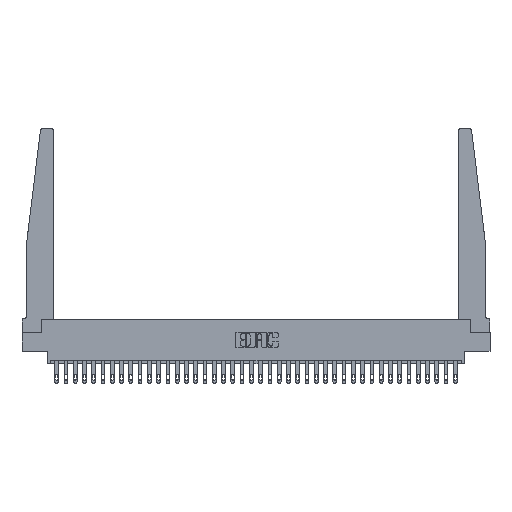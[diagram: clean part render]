
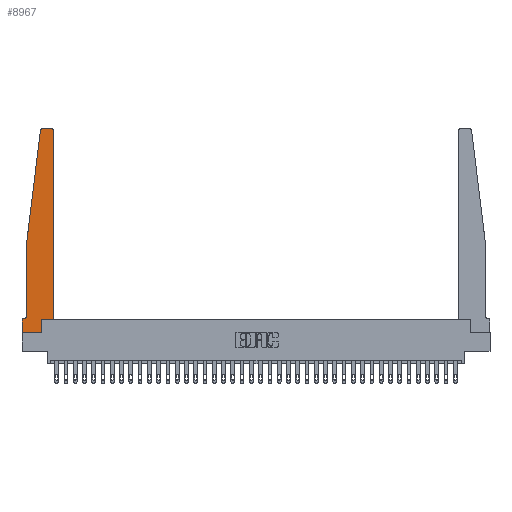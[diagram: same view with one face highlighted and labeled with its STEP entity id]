
A CAD part, top view. The second image highlights one B-rep face of the part: STEP entity #8967.
In plain terms, the highlighted planar face has unit normal (0, 0, 1).
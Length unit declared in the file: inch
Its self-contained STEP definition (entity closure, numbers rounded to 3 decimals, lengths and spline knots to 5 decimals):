
#457 = ORIENTED_EDGE ( 'NONE', *, *, #11465, .T. ) ;
#671 = ORIENTED_EDGE ( 'NONE', *, *, #31473, .T. ) ;
#787 = VERTEX_POINT ( 'NONE', #23877 ) ;
#1664 = VECTOR ( 'NONE', #19332, 39.37008 ) ;
#2096 = VERTEX_POINT ( 'NONE', #30226 ) ;
#2302 = DIRECTION ( 'NONE',  ( 1., 0., 0. ) ) ;
#2799 = DIRECTION ( 'NONE',  ( 0., 0., -1. ) ) ;
#3092 = LINE ( 'NONE', #8354, #9274 ) ;
#3141 = EDGE_CURVE ( 'NONE', #31485, #24207, #18799, .T. ) ;
#4517 = AXIS2_PLACEMENT_3D ( 'NONE', #7769, #13542, #21088 ) ;
#4764 = AXIS2_PLACEMENT_3D ( 'NONE', #23436, #2799, #31823 ) ;
#5004 = VECTOR ( 'NONE', #18298, 39.37008 ) ;
#5695 = EDGE_CURVE ( 'NONE', #9499, #8446, #24652, .T. ) ;
#5712 = VERTEX_POINT ( 'NONE', #26736 ) ;
#5932 = LINE ( 'NONE', #10493, #8910 ) ;
#6143 = VECTOR ( 'NONE', #16947, 39.37008 ) ;
#6240 = CARTESIAN_POINT ( 'NONE',  ( 0.065, 1.25, 0.37 ) ) ;
#6490 = LINE ( 'NONE', #16515, #27529 ) ;
#7472 = CARTESIAN_POINT ( 'NONE',  ( 0.25, 2.75, 0.37 ) ) ;
#7582 = LINE ( 'NONE', #13000, #5004 ) ;
#7655 = EDGE_CURVE ( 'NONE', #25096, #787, #6490, .T. ) ;
#7769 = CARTESIAN_POINT ( 'NONE',  ( 0.395, 2.72, 0.37 ) ) ;
#8354 = CARTESIAN_POINT ( 'NONE',  ( 0.065, 0.1875, 0.37 ) ) ;
#8446 = VERTEX_POINT ( 'NONE', #28793 ) ;
#8910 = VECTOR ( 'NONE', #31875, 39.37008 ) ;
#8967 = ADVANCED_FACE ( 'NONE', ( #17964 ), #18292, .T. ) ;
#9274 = VECTOR ( 'NONE', #31438, 39.37008 ) ;
#9285 = ORIENTED_EDGE ( 'NONE', *, *, #10119, .T. ) ;
#9445 = VERTEX_POINT ( 'NONE', #16657 ) ;
#9499 = VERTEX_POINT ( 'NONE', #13752 ) ;
#10119 = EDGE_CURVE ( 'NONE', #787, #9445, #27421, .T. ) ;
#10221 = VECTOR ( 'NONE', #29884, 39.37008 ) ;
#10323 = EDGE_CURVE ( 'NONE', #2096, #23289, #7582, .T. ) ;
#10493 = CARTESIAN_POINT ( 'NONE',  ( 0.425, 0.18, 0.37 ) ) ;
#11402 = DIRECTION ( 'NONE',  ( 0., 1., 0. ) ) ;
#11408 = CARTESIAN_POINT ( 'NONE',  ( 0.27653, 2.72, 0.37 ) ) ;
#11465 = EDGE_CURVE ( 'NONE', #9445, #9499, #5932, .T. ) ;
#11555 = ORIENTED_EDGE ( 'NONE', *, *, #19049, .T. ) ;
#12670 = CARTESIAN_POINT ( 'NONE',  ( 0., 0.1875, 0.37 ) ) ;
#12853 = CARTESIAN_POINT ( 'NONE',  ( 0.015, 0.1875, 0.37 ) ) ;
#13000 = CARTESIAN_POINT ( 'NONE',  ( 0., 0., 0.37 ) ) ;
#13542 = DIRECTION ( 'NONE',  ( 0., 0., 1. ) ) ;
#13752 = CARTESIAN_POINT ( 'NONE',  ( 0.425, 2.72, 0.37 ) ) ;
#13801 = ORIENTED_EDGE ( 'NONE', *, *, #7655, .T. ) ;
#15393 = DIRECTION ( 'NONE',  ( 0., 0., 1. ) ) ;
#16515 = CARTESIAN_POINT ( 'NONE',  ( 0.2605, 0.18, 0.37 ) ) ;
#16657 = CARTESIAN_POINT ( 'NONE',  ( 0.425, 0.18, 0.37 ) ) ;
#16676 = LINE ( 'NONE', #32425, #10221 ) ;
#16706 = ORIENTED_EDGE ( 'NONE', *, *, #20724, .T. ) ;
#16905 = CARTESIAN_POINT ( 'NONE',  ( 0.065, 1.25, 0.37 ) ) ;
#16947 = DIRECTION ( 'NONE',  ( 1., 0., 0. ) ) ;
#17964 = FACE_OUTER_BOUND ( 'NONE', #18062, .T. ) ;
#18062 = EDGE_LOOP ( 'NONE', ( #671, #16706, #25345, #11555, #26242, #21628, #30550, #21985, #13801, #9285, #457, #28156 ) ) ;
#18292 = PLANE ( 'NONE',  #26489 ) ;
#18298 = DIRECTION ( 'NONE',  ( 0., -1., 0. ) ) ;
#18457 = CARTESIAN_POINT ( 'NONE',  ( 0.065, 1.25, 0.37 ) ) ;
#18799 = LINE ( 'NONE', #18457, #25610 ) ;
#18996 = EDGE_CURVE ( 'NONE', #32122, #2096, #3092, .T. ) ;
#19049 = EDGE_CURVE ( 'NONE', #24207, #5712, #19832, .T. ) ;
#19332 = DIRECTION ( 'NONE',  ( 0., -1., 0. ) ) ;
#19832 = LINE ( 'NONE', #16905, #1664 ) ;
#19977 = DIRECTION ( 'NONE',  ( 1., 0., 0. ) ) ;
#20118 = DIRECTION ( 'NONE',  ( -1., 0., 0. ) ) ;
#20724 = EDGE_CURVE ( 'NONE', #27147, #31485, #32512, .T. ) ;
#21088 = DIRECTION ( 'NONE',  ( 1., 0., 0. ) ) ;
#21628 = ORIENTED_EDGE ( 'NONE', *, *, #18996, .T. ) ;
#21929 = EDGE_CURVE ( 'NONE', #5712, #32122, #29818, .T. ) ;
#21985 = ORIENTED_EDGE ( 'NONE', *, *, #31270, .T. ) ;
#22135 = AXIS2_PLACEMENT_3D ( 'NONE', #11408, #29910, #19977 ) ;
#23289 = VERTEX_POINT ( 'NONE', #23887 ) ;
#23436 = CARTESIAN_POINT ( 'NONE',  ( 0.015, 0.2375, 0.37 ) ) ;
#23877 = CARTESIAN_POINT ( 'NONE',  ( 0.2605, 0.18, 0.37 ) ) ;
#23887 = CARTESIAN_POINT ( 'NONE',  ( 0., 0., 0.37 ) ) ;
#24207 = VERTEX_POINT ( 'NONE', #6240 ) ;
#24652 = CIRCLE ( 'NONE', #4517, 0.03 ) ;
#25096 = VERTEX_POINT ( 'NONE', #29360 ) ;
#25345 = ORIENTED_EDGE ( 'NONE', *, *, #3141, .T. ) ;
#25610 = VECTOR ( 'NONE', #26170, 39.37008 ) ;
#26170 = DIRECTION ( 'NONE',  ( -0.122, -0.992, 0. ) ) ;
#26242 = ORIENTED_EDGE ( 'NONE', *, *, #21929, .T. ) ;
#26489 = AXIS2_PLACEMENT_3D ( 'NONE', #12670, #15393, #2302 ) ;
#26736 = CARTESIAN_POINT ( 'NONE',  ( 0.065, 0.2375, 0.37 ) ) ;
#27147 = VERTEX_POINT ( 'NONE', #28119 ) ;
#27421 = LINE ( 'NONE', #30320, #6143 ) ;
#27529 = VECTOR ( 'NONE', #11402, 39.37008 ) ;
#27649 = CARTESIAN_POINT ( 'NONE',  ( 0.24675, 2.72367, 0.37 ) ) ;
#28119 = CARTESIAN_POINT ( 'NONE',  ( 0.27653, 2.75, 0.37 ) ) ;
#28156 = ORIENTED_EDGE ( 'NONE', *, *, #5695, .T. ) ;
#28793 = CARTESIAN_POINT ( 'NONE',  ( 0.395, 2.75, 0.37 ) ) ;
#29360 = CARTESIAN_POINT ( 'NONE',  ( 0.2605, 0., 0.37 ) ) ;
#29818 = CIRCLE ( 'NONE', #4764, 0.05 ) ;
#29884 = DIRECTION ( 'NONE',  ( 1., 0., 0. ) ) ;
#29910 = DIRECTION ( 'NONE',  ( 0., 0., 1. ) ) ;
#30226 = CARTESIAN_POINT ( 'NONE',  ( 0., 0.1875, 0.37 ) ) ;
#30320 = CARTESIAN_POINT ( 'NONE',  ( 0.425, 0.18, 0.37 ) ) ;
#30550 = ORIENTED_EDGE ( 'NONE', *, *, #10323, .T. ) ;
#30881 = LINE ( 'NONE', #7472, #31549 ) ;
#31270 = EDGE_CURVE ( 'NONE', #23289, #25096, #16676, .T. ) ;
#31438 = DIRECTION ( 'NONE',  ( -1., 0., 0. ) ) ;
#31473 = EDGE_CURVE ( 'NONE', #8446, #27147, #30881, .T. ) ;
#31485 = VERTEX_POINT ( 'NONE', #27649 ) ;
#31549 = VECTOR ( 'NONE', #20118, 39.37008 ) ;
#31823 = DIRECTION ( 'NONE',  ( -1., 0., 0. ) ) ;
#31875 = DIRECTION ( 'NONE',  ( 0., 1., 0. ) ) ;
#32122 = VERTEX_POINT ( 'NONE', #12853 ) ;
#32425 = CARTESIAN_POINT ( 'NONE',  ( 0., 0., 0.37 ) ) ;
#32512 = CIRCLE ( 'NONE', #22135, 0.03 ) ;
